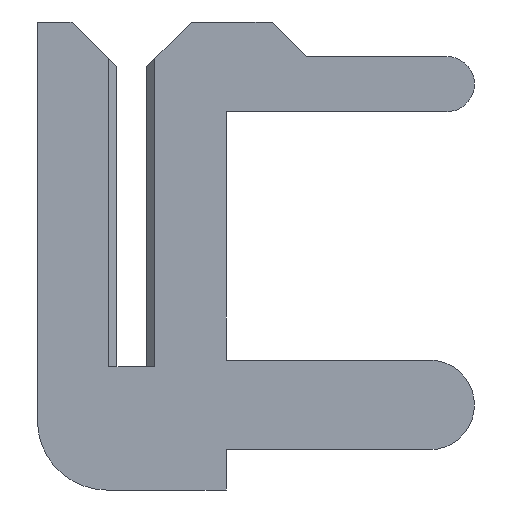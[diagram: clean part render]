
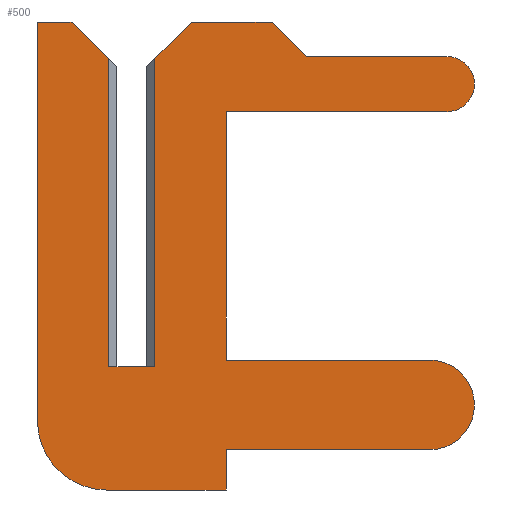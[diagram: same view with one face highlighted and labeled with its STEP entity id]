
A CAD part, left-side view. The second image highlights one B-rep face of the part: STEP entity #500.
In plain terms, the highlighted planar face has unit normal (-1, 0, 0).
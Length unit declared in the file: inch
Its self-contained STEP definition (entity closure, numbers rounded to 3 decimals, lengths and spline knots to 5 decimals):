
#2 = CARTESIAN_POINT ( 'NONE',  ( -0.01, -0.1295, 0.003 ) ) ;
#5 = DIRECTION ( 'NONE',  ( 0., 1., 0. ) ) ;
#13 = CARTESIAN_POINT ( 'NONE',  ( -0.01, -0.026, 0.15 ) ) ;
#14 = ORIENTED_EDGE ( 'NONE', *, *, #397, .F. ) ;
#15 = VECTOR ( 'NONE', #201, 39.37008 ) ;
#25 = CARTESIAN_POINT ( 'NONE',  ( -0.01, 0.011, -0.0235 ) ) ;
#27 = ORIENTED_EDGE ( 'NONE', *, *, #824, .F. ) ;
#33 = CARTESIAN_POINT ( 'NONE',  ( -0.01, -0.041, 0.003 ) ) ;
#41 = VECTOR ( 'NONE', #558, 39.37008 ) ;
#45 = LINE ( 'NONE', #904, #284 ) ;
#58 = VECTOR ( 'NONE', #175, 39.37008 ) ;
#61 = AXIS2_PLACEMENT_3D ( 'NONE', #518, #966, #794 ) ;
#71 = VERTEX_POINT ( 'NONE', #494 ) ;
#88 = EDGE_CURVE ( 'NONE', #873, #655, #565, .T. ) ;
#91 = CARTESIAN_POINT ( 'NONE',  ( -0.01, 0.01, 0. ) ) ;
#93 = DIRECTION ( 'NONE',  ( 0., -1., 0. ) ) ;
#95 = AXIS2_PLACEMENT_3D ( 'NONE', #25, #650, #752 ) ;
#99 = CARTESIAN_POINT ( 'NONE',  ( -0.01, -0.041, 0.111 ) ) ;
#108 = CARTESIAN_POINT ( 'NONE',  ( -0.01, 0.041, 0.15 ) ) ;
#123 = CARTESIAN_POINT ( 'NONE',  ( -0.01, -0.0065, 0.1305 ) ) ;
#124 = EDGE_CURVE ( 'NONE', #957, #71, #1022, .T. ) ;
#128 = LINE ( 'NONE', #108, #41 ) ;
#136 = CARTESIAN_POINT ( 'NONE',  ( -0.01, -0.076, 0.135 ) ) ;
#137 = LINE ( 'NONE', #123, #628 ) ;
#142 = LINE ( 'NONE', #1016, #15 ) ;
#158 = AXIS2_PLACEMENT_3D ( 'NONE', #203, #1024, #195 ) ;
#160 = CARTESIAN_POINT ( 'NONE',  ( -0.01, -0.041, -0.036 ) ) ;
#175 = DIRECTION ( 'NONE',  ( 0., -1., 0. ) ) ;
#191 = CARTESIAN_POINT ( 'NONE',  ( -0.01, -0.137, 0.123 ) ) ;
#193 = ORIENTED_EDGE ( 'NONE', *, *, #597, .F. ) ;
#195 = DIRECTION ( 'NONE',  ( 0., 0., 1. ) ) ;
#201 = DIRECTION ( 'NONE',  ( 0., 1., 0. ) ) ;
#203 = CARTESIAN_POINT ( 'NONE',  ( -0.01, 0.011, -0.0235 ) ) ;
#210 = VERTEX_POINT ( 'NONE', #160 ) ;
#218 = EDGE_CURVE ( 'NONE', #393, #334, #713, .T. ) ;
#219 = ORIENTED_EDGE ( 'NONE', *, *, #437, .F. ) ;
#228 = ORIENTED_EDGE ( 'NONE', *, *, #218, .F. ) ;
#241 = FACE_OUTER_BOUND ( 'NONE', #1004, .T. ) ;
#269 = LINE ( 'NONE', #360, #888 ) ;
#271 = ORIENTED_EDGE ( 'NONE', *, *, #682, .F. ) ;
#276 = CARTESIAN_POINT ( 'NONE',  ( -0.01, 0.026, 0.15 ) ) ;
#279 = DIRECTION ( 'NONE',  ( 0., 0., -1. ) ) ;
#284 = VECTOR ( 'NONE', #893, 39.37008 ) ;
#292 = DIRECTION ( 'NONE',  ( 0., 0., 1. ) ) ;
#299 = CARTESIAN_POINT ( 'NONE',  ( -0.01, -0.1295, -0.036 ) ) ;
#302 = EDGE_CURVE ( 'NONE', #831, #1069, #549, .T. ) ;
#308 = VECTOR ( 'NONE', #996, 39.37008 ) ;
#325 = CARTESIAN_POINT ( 'NONE',  ( -0.01, 0.026, 0.15 ) ) ;
#334 = VERTEX_POINT ( 'NONE', #276 ) ;
#342 = EDGE_CURVE ( 'NONE', #210, #957, #269, .T. ) ;
#345 = DIRECTION ( 'NONE',  ( 0., 1., 0. ) ) ;
#347 = DIRECTION ( 'NONE',  ( 0., 0., -1. ) ) ;
#353 = ORIENTED_EDGE ( 'NONE', *, *, #386, .F. ) ;
#357 = CARTESIAN_POINT ( 'NONE',  ( -0.01, -0.026, 0.15 ) ) ;
#360 = CARTESIAN_POINT ( 'NONE',  ( -0.01, -0.041, -0.0535 ) ) ;
#363 = CARTESIAN_POINT ( 'NONE',  ( -0.01, 0.0065, 0. ) ) ;
#377 = VECTOR ( 'NONE', #93, 39.37008 ) ;
#380 = LINE ( 'NONE', #533, #979 ) ;
#384 = PLANE ( 'NONE',  #158 ) ;
#385 = CARTESIAN_POINT ( 'NONE',  ( -0.01, 0.01, 0.134 ) ) ;
#386 = EDGE_CURVE ( 'NONE', #396, #1111, #801, .T. ) ;
#393 = VERTEX_POINT ( 'NONE', #920 ) ;
#396 = VERTEX_POINT ( 'NONE', #91 ) ;
#397 = EDGE_CURVE ( 'NONE', #1045, #799, #441, .T. ) ;
#405 = VECTOR ( 'NONE', #1157, 39.37008 ) ;
#414 = LINE ( 'NONE', #2, #377 ) ;
#417 = VECTOR ( 'NONE', #345, 39.37008 ) ;
#437 = EDGE_CURVE ( 'NONE', #334, #440, #45, .T. ) ;
#440 = VERTEX_POINT ( 'NONE', #385 ) ;
#441 = LINE ( 'NONE', #620, #308 ) ;
#450 = CARTESIAN_POINT ( 'NONE',  ( -0.01, -0.137, 0.135 ) ) ;
#454 = EDGE_CURVE ( 'NONE', #531, #963, #380, .T. ) ;
#494 = CARTESIAN_POINT ( 'NONE',  ( -0.01, 0.011, -0.0535 ) ) ;
#500 = ADVANCED_FACE ( 'NONE', ( #241 ), #384, .T. ) ;
#501 = VERTEX_POINT ( 'NONE', #739 ) ;
#518 = CARTESIAN_POINT ( 'NONE',  ( -0.01, -0.1295, -0.0165 ) ) ;
#531 = VERTEX_POINT ( 'NONE', #99 ) ;
#533 = CARTESIAN_POINT ( 'NONE',  ( -0.01, -0.041, 0.003 ) ) ;
#546 = LINE ( 'NONE', #734, #560 ) ;
#549 = LINE ( 'NONE', #357, #58 ) ;
#556 = CARTESIAN_POINT ( 'NONE',  ( -0.01, -0.01, 0.134 ) ) ;
#557 = DIRECTION ( 'NONE',  ( 1., 0., 0. ) ) ;
#558 = DIRECTION ( 'NONE',  ( 0., 0., 1. ) ) ;
#560 = VECTOR ( 'NONE', #5, 39.37008 ) ;
#565 = CIRCLE ( 'NONE', #61, 0.0195 ) ;
#571 = EDGE_CURVE ( 'NONE', #889, #1111, #644, .T. ) ;
#584 = EDGE_CURVE ( 'NONE', #501, #531, #142, .T. ) ;
#589 = ORIENTED_EDGE ( 'NONE', *, *, #302, .F. ) ;
#591 = DIRECTION ( 'NONE',  ( 0., -0.707, -0.707 ) ) ;
#597 = EDGE_CURVE ( 'NONE', #799, #501, #671, .T. ) ;
#620 = CARTESIAN_POINT ( 'NONE',  ( -0.01, -0.137, 0.135 ) ) ;
#621 = AXIS2_PLACEMENT_3D ( 'NONE', #191, #557, #292 ) ;
#628 = VECTOR ( 'NONE', #1030, 39.37008 ) ;
#637 = DIRECTION ( 'NONE',  ( 0., 0., -1. ) ) ;
#641 = VECTOR ( 'NONE', #1031, 39.37008 ) ;
#644 = LINE ( 'NONE', #821, #947 ) ;
#650 = DIRECTION ( 'NONE',  ( 1., 0., 0. ) ) ;
#653 = EDGE_CURVE ( 'NONE', #396, #440, #1032, .T. ) ;
#655 = VERTEX_POINT ( 'NONE', #299 ) ;
#671 = CIRCLE ( 'NONE', #621, 0.012 ) ;
#675 = CARTESIAN_POINT ( 'NONE',  ( -0.01, -0.061, 0.15 ) ) ;
#682 = EDGE_CURVE ( 'NONE', #71, #916, #1108, .T. ) ;
#713 = LINE ( 'NONE', #325, #1046 ) ;
#727 = ORIENTED_EDGE ( 'NONE', *, *, #342, .F. ) ;
#734 = CARTESIAN_POINT ( 'NONE',  ( -0.01, -0.041, -0.036 ) ) ;
#738 = CARTESIAN_POINT ( 'NONE',  ( -0.01, -0.1295, 0.003 ) ) ;
#739 = CARTESIAN_POINT ( 'NONE',  ( -0.01, -0.137, 0.111 ) ) ;
#750 = CARTESIAN_POINT ( 'NONE',  ( -0.01, 0.01, -0.0235 ) ) ;
#752 = DIRECTION ( 'NONE',  ( 0., 0., 1. ) ) ;
#788 = ORIENTED_EDGE ( 'NONE', *, *, #807, .F. ) ;
#794 = DIRECTION ( 'NONE',  ( 0., 0., 1. ) ) ;
#799 = VERTEX_POINT ( 'NONE', #450 ) ;
#801 = LINE ( 'NONE', #363, #405 ) ;
#807 = EDGE_CURVE ( 'NONE', #916, #393, #128, .T. ) ;
#813 = VECTOR ( 'NONE', #591, 39.37008 ) ;
#821 = CARTESIAN_POINT ( 'NONE',  ( -0.01, -0.01, 0.15 ) ) ;
#824 = EDGE_CURVE ( 'NONE', #655, #210, #546, .T. ) ;
#831 = VERTEX_POINT ( 'NONE', #13 ) ;
#847 = ORIENTED_EDGE ( 'NONE', *, *, #124, .F. ) ;
#861 = ORIENTED_EDGE ( 'NONE', *, *, #571, .T. ) ;
#863 = ORIENTED_EDGE ( 'NONE', *, *, #970, .F. ) ;
#873 = VERTEX_POINT ( 'NONE', #738 ) ;
#887 = ORIENTED_EDGE ( 'NONE', *, *, #1020, .F. ) ;
#888 = VECTOR ( 'NONE', #347, 39.37008 ) ;
#889 = VERTEX_POINT ( 'NONE', #556 ) ;
#893 = DIRECTION ( 'NONE',  ( 0., -0.707, -0.707 ) ) ;
#904 = CARTESIAN_POINT ( 'NONE',  ( -0.01, 0.0065, 0.1305 ) ) ;
#909 = EDGE_CURVE ( 'NONE', #963, #873, #414, .T. ) ;
#916 = VERTEX_POINT ( 'NONE', #1001 ) ;
#920 = CARTESIAN_POINT ( 'NONE',  ( -0.01, 0.041, 0.15 ) ) ;
#940 = CARTESIAN_POINT ( 'NONE',  ( -0.01, -0.041, -0.0535 ) ) ;
#947 = VECTOR ( 'NONE', #279, 39.37008 ) ;
#949 = ORIENTED_EDGE ( 'NONE', *, *, #88, .F. ) ;
#957 = VERTEX_POINT ( 'NONE', #940 ) ;
#963 = VERTEX_POINT ( 'NONE', #33 ) ;
#966 = DIRECTION ( 'NONE',  ( 1., 0., 0. ) ) ;
#970 = EDGE_CURVE ( 'NONE', #889, #831, #137, .T. ) ;
#978 = ORIENTED_EDGE ( 'NONE', *, *, #584, .F. ) ;
#979 = VECTOR ( 'NONE', #637, 39.37008 ) ;
#996 = DIRECTION ( 'NONE',  ( 0., -1., 0. ) ) ;
#1001 = CARTESIAN_POINT ( 'NONE',  ( -0.01, 0.041, -0.0235 ) ) ;
#1004 = EDGE_LOOP ( 'NONE', ( #863, #861, #353, #1123, #219, #228, #788, #271, #847, #727, #27, #949, #1127, #1060, #978, #193, #14, #887, #589 ) ) ;
#1015 = CARTESIAN_POINT ( 'NONE',  ( -0.01, -0.076, 0.135 ) ) ;
#1016 = CARTESIAN_POINT ( 'NONE',  ( -0.01, -0.041, 0.111 ) ) ;
#1020 = EDGE_CURVE ( 'NONE', #1069, #1045, #1058, .T. ) ;
#1022 = LINE ( 'NONE', #1142, #417 ) ;
#1024 = DIRECTION ( 'NONE',  ( -1., 0., 0. ) ) ;
#1030 = DIRECTION ( 'NONE',  ( 0., -0.707, 0.707 ) ) ;
#1031 = DIRECTION ( 'NONE',  ( 0., 0., 1. ) ) ;
#1032 = LINE ( 'NONE', #750, #641 ) ;
#1045 = VERTEX_POINT ( 'NONE', #136 ) ;
#1046 = VECTOR ( 'NONE', #1066, 39.37008 ) ;
#1050 = CARTESIAN_POINT ( 'NONE',  ( -0.01, -0.01, 0. ) ) ;
#1058 = LINE ( 'NONE', #1015, #813 ) ;
#1060 = ORIENTED_EDGE ( 'NONE', *, *, #454, .F. ) ;
#1066 = DIRECTION ( 'NONE',  ( 0., -1., 0. ) ) ;
#1069 = VERTEX_POINT ( 'NONE', #675 ) ;
#1108 = CIRCLE ( 'NONE', #95, 0.03 ) ;
#1111 = VERTEX_POINT ( 'NONE', #1050 ) ;
#1123 = ORIENTED_EDGE ( 'NONE', *, *, #653, .T. ) ;
#1127 = ORIENTED_EDGE ( 'NONE', *, *, #909, .F. ) ;
#1142 = CARTESIAN_POINT ( 'NONE',  ( -0.01, 0.011, -0.0535 ) ) ;
#1157 = DIRECTION ( 'NONE',  ( 0., -1., 0. ) ) ;
